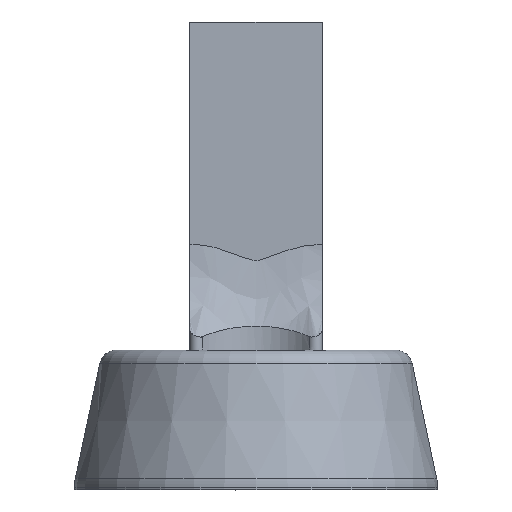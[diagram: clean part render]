
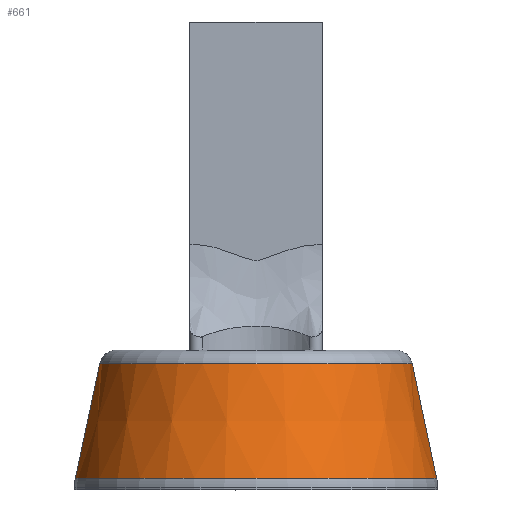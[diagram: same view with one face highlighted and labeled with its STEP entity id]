
A CAD part, front view. The second image highlights one B-rep face of the part: STEP entity #661.
In plain terms, the highlighted conical face has half-angle 12 degrees and reference radius 12.065 mm.
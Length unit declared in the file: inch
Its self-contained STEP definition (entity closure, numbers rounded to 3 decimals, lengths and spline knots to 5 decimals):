
#17=CONICAL_SURFACE('',#760,0.475,0.209);
#76=CIRCLE('',#741,0.44342);
#86=CIRCLE('',#759,0.51227);
#118=LINE('',#1559,#160);
#123=LINE('',#1581,#165);
#160=VECTOR('',#922,0.3937);
#165=VECTOR('',#951,0.3937);
#216=FACE_OUTER_BOUND('',#261,.T.);
#261=EDGE_LOOP('',(#600,#601,#602,#603));
#329=VERTEX_POINT('',#1538);
#330=VERTEX_POINT('',#1542);
#334=VERTEX_POINT('',#1558);
#339=VERTEX_POINT('',#1574);
#411=EDGE_CURVE('',#330,#329,#76,.T.);
#418=EDGE_CURVE('',#329,#334,#118,.T.);
#429=EDGE_CURVE('',#334,#339,#86,.T.);
#430=EDGE_CURVE('',#330,#339,#123,.T.);
#600=ORIENTED_EDGE('',*,*,#411,.F.);
#601=ORIENTED_EDGE('',*,*,#430,.T.);
#602=ORIENTED_EDGE('',*,*,#429,.F.);
#603=ORIENTED_EDGE('',*,*,#418,.F.);
#661=ADVANCED_FACE('',(#216),#17,.T.);
#741=AXIS2_PLACEMENT_3D('',#1544,#903,#904);
#759=AXIS2_PLACEMENT_3D('',#1579,#947,#948);
#760=AXIS2_PLACEMENT_3D('',#1580,#949,#950);
#903=DIRECTION('center_axis',(0.,0.,1.));
#904=DIRECTION('ref_axis',(0.,-1.,0.));
#922=DIRECTION('',(0.208,0.,-0.978));
#947=DIRECTION('center_axis',(0.,0.,
-1.));
#948=DIRECTION('ref_axis',(0.,-1.,0.));
#949=DIRECTION('center_axis',(0.,0.,-1.));
#950=DIRECTION('ref_axis',(1.,0.,0.));
#951=DIRECTION('',(-0.208,0.,-0.978));
#1538=CARTESIAN_POINT('',(-0.30201,-2.55,0.35725));
#1542=CARTESIAN_POINT('',(-1.18884,-2.55,0.35725));
#1544=CARTESIAN_POINT('Origin',(-0.74542,-2.55,0.35725));
#1558=CARTESIAN_POINT('',(-0.23316,-2.55,0.03333));
#1559=CARTESIAN_POINT('',(-0.31042,-2.55,0.39685));
#1574=CARTESIAN_POINT('',(-1.25769,-2.55,0.03333));
#1579=CARTESIAN_POINT('Origin',(-0.74542,-2.55,0.03333));
#1580=CARTESIAN_POINT('Origin',(-0.74542,-2.55,0.20867));
#1581=CARTESIAN_POINT('',(-1.18042,-2.55,0.39685));
